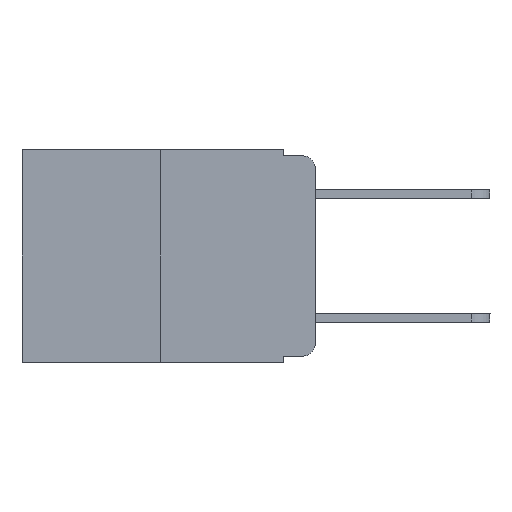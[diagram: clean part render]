
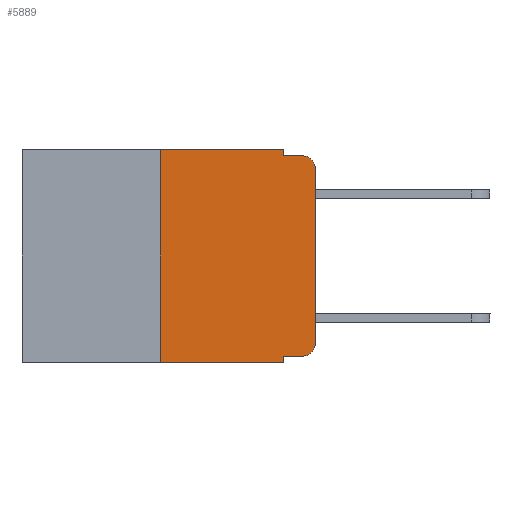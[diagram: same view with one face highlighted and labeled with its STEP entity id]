
A CAD part, left-side view. The second image highlights one B-rep face of the part: STEP entity #5889.
In plain terms, the highlighted planar face has unit normal (-1, 0, 0).
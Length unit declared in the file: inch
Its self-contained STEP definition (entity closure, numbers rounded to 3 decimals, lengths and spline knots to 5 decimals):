
#762 = DIRECTION ( 'NONE',  ( 0., 0., -1. ) ) ;
#779 = VECTOR ( 'NONE', #20513, 39.37008 ) ;
#908 = VERTEX_POINT ( 'NONE', #12796 ) ;
#937 = ORIENTED_EDGE ( 'NONE', *, *, #9156, .T. ) ;
#991 = VECTOR ( 'NONE', #14306, 39.37008 ) ;
#1046 = VERTEX_POINT ( 'NONE', #10139 ) ;
#1057 = DIRECTION ( 'NONE',  ( -1., 0., 0. ) ) ;
#1820 = CARTESIAN_POINT ( 'NONE',  ( 0., 0.051, 0. ) ) ;
#2273 = CIRCLE ( 'NONE', #4987, 0.02 ) ;
#2305 = EDGE_CURVE ( 'NONE', #14541, #1046, #6104, .T. ) ;
#2467 = DIRECTION ( 'NONE',  ( 0., 0., -1. ) ) ;
#2473 = EDGE_CURVE ( 'NONE', #3550, #3796, #14132, .T. ) ;
#2510 = VECTOR ( 'NONE', #15144, 39.37008 ) ;
#2572 = DIRECTION ( 'NONE',  ( 0., 0., 1. ) ) ;
#2808 = CARTESIAN_POINT ( 'NONE',  ( 0., 0.051, -0.333 ) ) ;
#2931 = AXIS2_PLACEMENT_3D ( 'NONE', #7224, #19962, #6950 ) ;
#3550 = VERTEX_POINT ( 'NONE', #12252 ) ;
#3576 = EDGE_CURVE ( 'NONE', #20847, #11719, #10423, .T. ) ;
#3796 = VERTEX_POINT ( 'NONE', #10923 ) ;
#3805 = CARTESIAN_POINT ( 'NONE',  ( 0., 0.051, -0.01 ) ) ;
#3862 = CARTESIAN_POINT ( 'NONE',  ( 0., 0.051, 0. ) ) ;
#4107 = CARTESIAN_POINT ( 'NONE',  ( 0., 0.051, -0.01 ) ) ;
#4270 = ORIENTED_EDGE ( 'NONE', *, *, #18051, .F. ) ;
#4886 = EDGE_CURVE ( 'NONE', #20847, #908, #14410, .T. ) ;
#4987 = AXIS2_PLACEMENT_3D ( 'NONE', #18656, #1057, #2467 ) ;
#5409 = DIRECTION ( 'NONE',  ( 0., -1., 0. ) ) ;
#5633 = DIRECTION ( 'NONE',  ( 1., 0., 0. ) ) ;
#5709 = CARTESIAN_POINT ( 'NONE',  ( 0., 0.25, 0. ) ) ;
#5859 = EDGE_LOOP ( 'NONE', ( #7295, #937, #7832, #6936, #11144, #6663, #7478, #4270, #10907, #6784 ) ) ;
#5889 = ADVANCED_FACE ( 'NONE', ( #18627 ), #20075, .F. ) ;
#6019 = EDGE_CURVE ( 'NONE', #3796, #14541, #2273, .T. ) ;
#6104 = LINE ( 'NONE', #7084, #11403 ) ;
#6663 = ORIENTED_EDGE ( 'NONE', *, *, #3576, .F. ) ;
#6784 = ORIENTED_EDGE ( 'NONE', *, *, #6019, .T. ) ;
#6936 = ORIENTED_EDGE ( 'NONE', *, *, #20280, .F. ) ;
#6950 = DIRECTION ( 'NONE',  ( 0., 0., -1. ) ) ;
#7084 = CARTESIAN_POINT ( 'NONE',  ( 0., 0., 0. ) ) ;
#7224 = CARTESIAN_POINT ( 'NONE',  ( 0., 0.02, -0.03 ) ) ;
#7295 = ORIENTED_EDGE ( 'NONE', *, *, #2305, .T. ) ;
#7478 = ORIENTED_EDGE ( 'NONE', *, *, #4886, .T. ) ;
#7559 = LINE ( 'NONE', #9605, #991 ) ;
#7832 = ORIENTED_EDGE ( 'NONE', *, *, #14193, .F. ) ;
#7892 = VECTOR ( 'NONE', #2572, 39.37008 ) ;
#8092 = DIRECTION ( 'NONE',  ( 0., 0., -1. ) ) ;
#9156 = EDGE_CURVE ( 'NONE', #1046, #17347, #13954, .T. ) ;
#9605 = CARTESIAN_POINT ( 'NONE',  ( 0., 0.051, 0. ) ) ;
#10139 = CARTESIAN_POINT ( 'NONE',  ( 0., 0., -0.03 ) ) ;
#10423 = LINE ( 'NONE', #10623, #7892 ) ;
#10623 = CARTESIAN_POINT ( 'NONE',  ( 0., 0.25, 0. ) ) ;
#10757 = CARTESIAN_POINT ( 'NONE',  ( 0., 0.02, -0.01 ) ) ;
#10907 = ORIENTED_EDGE ( 'NONE', *, *, #2473, .T. ) ;
#10923 = CARTESIAN_POINT ( 'NONE',  ( 0., 0.02, -0.333 ) ) ;
#11144 = ORIENTED_EDGE ( 'NONE', *, *, #17148, .F. ) ;
#11403 = VECTOR ( 'NONE', #18318, 39.37008 ) ;
#11719 = VERTEX_POINT ( 'NONE', #5709 ) ;
#11836 = CARTESIAN_POINT ( 'NONE',  ( 0., 0.473, 0. ) ) ;
#12252 = CARTESIAN_POINT ( 'NONE',  ( 0., 0.051, -0.333 ) ) ;
#12457 = VERTEX_POINT ( 'NONE', #4107 ) ;
#12796 = CARTESIAN_POINT ( 'NONE',  ( 0., 0.051, -0.343 ) ) ;
#13113 = CARTESIAN_POINT ( 'NONE',  ( 0., 0.473, 0. ) ) ;
#13743 = AXIS2_PLACEMENT_3D ( 'NONE', #13113, #5633, #762 ) ;
#13954 = CIRCLE ( 'NONE', #2931, 0.02 ) ;
#14132 = LINE ( 'NONE', #2808, #779 ) ;
#14193 = EDGE_CURVE ( 'NONE', #12457, #17347, #15100, .T. ) ;
#14306 = DIRECTION ( 'NONE',  ( 0., 0., -1. ) ) ;
#14410 = LINE ( 'NONE', #15450, #18180 ) ;
#14541 = VERTEX_POINT ( 'NONE', #20788 ) ;
#14741 = LINE ( 'NONE', #1820, #18531 ) ;
#15100 = LINE ( 'NONE', #3805, #2510 ) ;
#15144 = DIRECTION ( 'NONE',  ( 0., -1., 0. ) ) ;
#15450 = CARTESIAN_POINT ( 'NONE',  ( 0., 0.473, -0.343 ) ) ;
#17148 = EDGE_CURVE ( 'NONE', #11719, #18408, #20661, .T. ) ;
#17347 = VERTEX_POINT ( 'NONE', #10757 ) ;
#17697 = CARTESIAN_POINT ( 'NONE',  ( 0., 0.25, -0.343 ) ) ;
#18051 = EDGE_CURVE ( 'NONE', #3550, #908, #7559, .T. ) ;
#18180 = VECTOR ( 'NONE', #18971, 39.37008 ) ;
#18318 = DIRECTION ( 'NONE',  ( 0., 0., 1. ) ) ;
#18408 = VERTEX_POINT ( 'NONE', #3862 ) ;
#18531 = VECTOR ( 'NONE', #8092, 39.37008 ) ;
#18627 = FACE_OUTER_BOUND ( 'NONE', #5859, .T. ) ;
#18656 = CARTESIAN_POINT ( 'NONE',  ( 0., 0.02, -0.313 ) ) ;
#18971 = DIRECTION ( 'NONE',  ( 0., -1., 0. ) ) ;
#19962 = DIRECTION ( 'NONE',  ( -1., 0., 0. ) ) ;
#20075 = PLANE ( 'NONE',  #13743 ) ;
#20280 = EDGE_CURVE ( 'NONE', #18408, #12457, #14741, .T. ) ;
#20406 = VECTOR ( 'NONE', #5409, 39.37008 ) ;
#20513 = DIRECTION ( 'NONE',  ( 0., -1., 0. ) ) ;
#20661 = LINE ( 'NONE', #11836, #20406 ) ;
#20788 = CARTESIAN_POINT ( 'NONE',  ( 0., 0., -0.313 ) ) ;
#20847 = VERTEX_POINT ( 'NONE', #17697 ) ;
